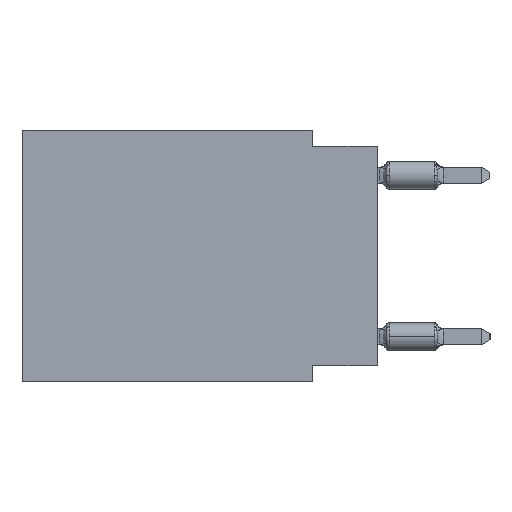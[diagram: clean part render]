
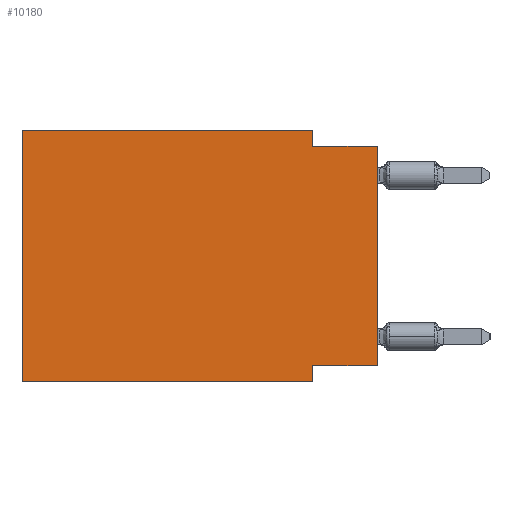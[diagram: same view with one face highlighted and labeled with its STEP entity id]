
A CAD part, left-side view. The second image highlights one B-rep face of the part: STEP entity #10180.
In plain terms, the highlighted planar face has unit normal (-1, 0, 0).
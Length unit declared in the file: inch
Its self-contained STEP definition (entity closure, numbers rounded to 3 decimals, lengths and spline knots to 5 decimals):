
#257 = ORIENTED_EDGE ( 'NONE', *, *, #33974, .F. ) ;
#1405 = EDGE_CURVE ( 'NONE', #3827, #4890, #14171, .T. ) ;
#3723 = VECTOR ( 'NONE', #6892, 39.37008 ) ;
#3812 = CARTESIAN_POINT ( 'NONE',  ( 0., 0.1, -0.025 ) ) ;
#3827 = VERTEX_POINT ( 'NONE', #3812 ) ;
#4183 = CARTESIAN_POINT ( 'NONE',  ( 0., 0., -0.025 ) ) ;
#4583 = LINE ( 'NONE', #25734, #45917 ) ;
#4890 = VERTEX_POINT ( 'NONE', #4183 ) ;
#5847 = DIRECTION ( 'NONE',  ( 0., -1., 0. ) ) ;
#6892 = DIRECTION ( 'NONE',  ( 0., 0., -1. ) ) ;
#7170 = PLANE ( 'NONE',  #21183 ) ;
#8424 = ORIENTED_EDGE ( 'NONE', *, *, #21429, .F. ) ;
#9359 = CARTESIAN_POINT ( 'NONE',  ( 0., 0.1, 0. ) ) ;
#9463 = DIRECTION ( 'NONE',  ( 0., -1., 0. ) ) ;
#10180 = ADVANCED_FACE ( 'NONE', ( #29059 ), #7170, .F. ) ;
#10199 = ORIENTED_EDGE ( 'NONE', *, *, #14415, .T. ) ;
#10531 = CARTESIAN_POINT ( 'NONE',  ( 0., 0., -0.025 ) ) ;
#10898 = DIRECTION ( 'NONE',  ( 0., 1., 0. ) ) ;
#11544 = CARTESIAN_POINT ( 'NONE',  ( 0., 0.1, -0.39 ) ) ;
#11762 = ORIENTED_EDGE ( 'NONE', *, *, #47140, .F. ) ;
#13602 = LINE ( 'NONE', #28446, #16191 ) ;
#14150 = LINE ( 'NONE', #47179, #31197 ) ;
#14171 = LINE ( 'NONE', #10531, #18049 ) ;
#14415 = EDGE_CURVE ( 'NONE', #29692, #31222, #46366, .T. ) ;
#14463 = DIRECTION ( 'NONE',  ( 1., 0., 0. ) ) ;
#14529 = VECTOR ( 'NONE', #36186, 39.37008 ) ;
#16191 = VECTOR ( 'NONE', #5847, 39.37008 ) ;
#16987 = EDGE_LOOP ( 'NONE', ( #18734, #38149, #41375, #257, #8424, #10199, #18851, #11762 ) ) ;
#17491 = CARTESIAN_POINT ( 'NONE',  ( 0., 0.55, 0. ) ) ;
#17972 = LINE ( 'NONE', #17491, #14529 ) ;
#18049 = VECTOR ( 'NONE', #40149, 39.37008 ) ;
#18734 = ORIENTED_EDGE ( 'NONE', *, *, #38022, .T. ) ;
#18851 = ORIENTED_EDGE ( 'NONE', *, *, #33251, .F. ) ;
#19076 = CARTESIAN_POINT ( 'NONE',  ( 0., 0.1, -0.365 ) ) ;
#19424 = DIRECTION ( 'NONE',  ( 0., 0., -1. ) ) ;
#21183 = AXIS2_PLACEMENT_3D ( 'NONE', #25405, #14463, #47478 ) ;
#21429 = EDGE_CURVE ( 'NONE', #29692, #36067, #17972, .T. ) ;
#21476 = LINE ( 'NONE', #24185, #3723 ) ;
#22525 = CARTESIAN_POINT ( 'NONE',  ( 0., 0.55, 0. ) ) ;
#24179 = VERTEX_POINT ( 'NONE', #32778 ) ;
#24185 = CARTESIAN_POINT ( 'NONE',  ( 0., 0.1, -0.39 ) ) ;
#24417 = VECTOR ( 'NONE', #9463, 39.37008 ) ;
#25405 = CARTESIAN_POINT ( 'NONE',  ( 0., 0.55, 0. ) ) ;
#25734 = CARTESIAN_POINT ( 'NONE',  ( 0., 0.1, 0. ) ) ;
#26325 = VERTEX_POINT ( 'NONE', #19076 ) ;
#28446 = CARTESIAN_POINT ( 'NONE',  ( 0., 0.55, 0. ) ) ;
#28991 = DIRECTION ( 'NONE',  ( 0., 0., 1. ) ) ;
#29059 = FACE_OUTER_BOUND ( 'NONE', #16987, .T. ) ;
#29385 = CARTESIAN_POINT ( 'NONE',  ( 0., 0., -0.365 ) ) ;
#29692 = VERTEX_POINT ( 'NONE', #47718 ) ;
#31197 = VECTOR ( 'NONE', #28991, 39.37008 ) ;
#31222 = VERTEX_POINT ( 'NONE', #11544 ) ;
#31998 = VERTEX_POINT ( 'NONE', #9359 ) ;
#32778 = CARTESIAN_POINT ( 'NONE',  ( 0., 0., -0.365 ) ) ;
#33251 = EDGE_CURVE ( 'NONE', #26325, #31222, #21476, .T. ) ;
#33974 = EDGE_CURVE ( 'NONE', #36067, #31998, #13602, .T. ) ;
#35907 = CARTESIAN_POINT ( 'NONE',  ( 0., 0.55, -0.39 ) ) ;
#36067 = VERTEX_POINT ( 'NONE', #22525 ) ;
#36186 = DIRECTION ( 'NONE',  ( 0., 0., 1. ) ) ;
#38022 = EDGE_CURVE ( 'NONE', #24179, #4890, #14150, .T. ) ;
#38149 = ORIENTED_EDGE ( 'NONE', *, *, #1405, .F. ) ;
#40149 = DIRECTION ( 'NONE',  ( 0., -1., 0. ) ) ;
#41375 = ORIENTED_EDGE ( 'NONE', *, *, #47100, .F. ) ;
#44162 = LINE ( 'NONE', #29385, #47449 ) ;
#45917 = VECTOR ( 'NONE', #19424, 39.37008 ) ;
#46366 = LINE ( 'NONE', #35907, #24417 ) ;
#47100 = EDGE_CURVE ( 'NONE', #31998, #3827, #4583, .T. ) ;
#47140 = EDGE_CURVE ( 'NONE', #24179, #26325, #44162, .T. ) ;
#47179 = CARTESIAN_POINT ( 'NONE',  ( 0., 0., 0. ) ) ;
#47449 = VECTOR ( 'NONE', #10898, 39.37008 ) ;
#47478 = DIRECTION ( 'NONE',  ( 0., 0., -1. ) ) ;
#47718 = CARTESIAN_POINT ( 'NONE',  ( 0., 0.55, -0.39 ) ) ;
